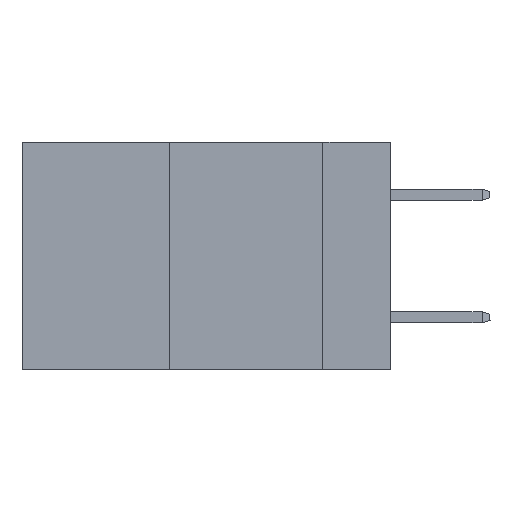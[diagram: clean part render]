
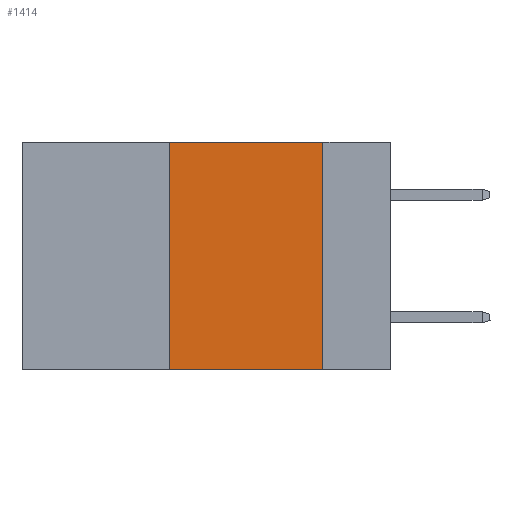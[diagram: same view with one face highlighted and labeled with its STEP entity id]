
A CAD part, left-side view. The second image highlights one B-rep face of the part: STEP entity #1414.
In plain terms, the highlighted planar face has unit normal (-1, 0, 0).
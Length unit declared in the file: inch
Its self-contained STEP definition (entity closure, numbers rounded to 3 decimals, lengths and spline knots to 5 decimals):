
#246 = CARTESIAN_POINT ( 'NONE',  ( 0., 0.11, -0.37 ) ) ;
#1414 = ADVANCED_FACE ( 'NONE', ( #21544 ), #2811, .F. ) ;
#1929 = VECTOR ( 'NONE', #7409, 39.37008 ) ;
#2703 = CARTESIAN_POINT ( 'NONE',  ( 0., 0.36, -0.37 ) ) ;
#2811 = PLANE ( 'NONE',  #3669 ) ;
#2975 = EDGE_CURVE ( 'NONE', #12982, #5787, #11615, .T. ) ;
#3669 = AXIS2_PLACEMENT_3D ( 'NONE', #21601, #23642, #13240 ) ;
#4173 = ORIENTED_EDGE ( 'NONE', *, *, #2975, .F. ) ;
#4716 = DIRECTION ( 'NONE',  ( 0., -1., 0. ) ) ;
#5347 = VECTOR ( 'NONE', #10244, 39.37008 ) ;
#5787 = VERTEX_POINT ( 'NONE', #22597 ) ;
#6627 = CARTESIAN_POINT ( 'NONE',  ( 0., 0.6, -0.37 ) ) ;
#7273 = LINE ( 'NONE', #15863, #1929 ) ;
#7409 = DIRECTION ( 'NONE',  ( 0., 0., -1. ) ) ;
#8083 = EDGE_CURVE ( 'NONE', #10103, #24680, #7273, .T. ) ;
#8349 = ORIENTED_EDGE ( 'NONE', *, *, #13828, .T. ) ;
#8429 = EDGE_LOOP ( 'NONE', ( #10547, #22956, #4173, #8349 ) ) ;
#8802 = VECTOR ( 'NONE', #4716, 39.37008 ) ;
#9012 = DIRECTION ( 'NONE',  ( 0., -1., 0. ) ) ;
#10103 = VERTEX_POINT ( 'NONE', #10640 ) ;
#10244 = DIRECTION ( 'NONE',  ( 0., 0., 1. ) ) ;
#10547 = ORIENTED_EDGE ( 'NONE', *, *, #8083, .F. ) ;
#10640 = CARTESIAN_POINT ( 'NONE',  ( 0., 0.11, 0. ) ) ;
#11615 = LINE ( 'NONE', #22850, #5347 ) ;
#12973 = EDGE_CURVE ( 'NONE', #5787, #10103, #15372, .T. ) ;
#12982 = VERTEX_POINT ( 'NONE', #2703 ) ;
#13240 = DIRECTION ( 'NONE',  ( 0., 0., -1. ) ) ;
#13828 = EDGE_CURVE ( 'NONE', #12982, #24680, #25531, .T. ) ;
#15372 = LINE ( 'NONE', #15711, #8802 ) ;
#15711 = CARTESIAN_POINT ( 'NONE',  ( 0., 0.6, 0. ) ) ;
#15863 = CARTESIAN_POINT ( 'NONE',  ( 0., 0.11, 0. ) ) ;
#19915 = VECTOR ( 'NONE', #9012, 39.37008 ) ;
#21544 = FACE_OUTER_BOUND ( 'NONE', #8429, .T. ) ;
#21601 = CARTESIAN_POINT ( 'NONE',  ( 0., 0.6, 0. ) ) ;
#22597 = CARTESIAN_POINT ( 'NONE',  ( 0., 0.36, 0. ) ) ;
#22850 = CARTESIAN_POINT ( 'NONE',  ( 0., 0.36, 0. ) ) ;
#22956 = ORIENTED_EDGE ( 'NONE', *, *, #12973, .F. ) ;
#23642 = DIRECTION ( 'NONE',  ( 1., 0., 0. ) ) ;
#24680 = VERTEX_POINT ( 'NONE', #246 ) ;
#25531 = LINE ( 'NONE', #6627, #19915 ) ;
